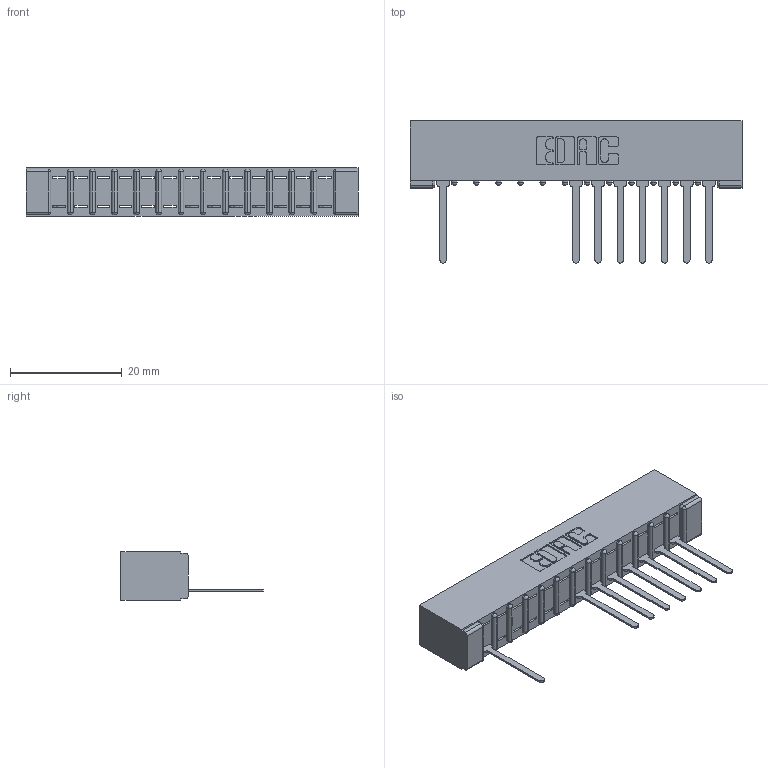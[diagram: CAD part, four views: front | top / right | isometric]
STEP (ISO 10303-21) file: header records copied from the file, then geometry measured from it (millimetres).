
FILE_DESCRIPTION (( 'STEP AP203' ), '1' );
FILE_NAME ('357-013-547-101.STEP', '2018-08-07T22:45:16', ( '' ), ( '' ), 'SwSTEP 2.0', 'SolidWorks 2016', '' );
FILE_SCHEMA (( 'CONFIG_CONTROL_DESIGN' ));
Length unit declared in the file: inch
Products named in the file (3): 307-290-001_547; 357-013-547-101; 307 Part_No Mounting Lugs
Assembly tree (9 placements, depth 2):
  357-013-547-101
    307 Part_No Mounting Lugs
    307-290-001_547  x8
Bounding box: 59.39 x 25.43 x 8.71 mm (x, y, z)
Volume: 3916.4 mm3; surface area: 5715 mm2
Topology: 9 solids, 9 shells, 672 faces, 1915 edges, 1226 vertices
Faces by surface type: plane 422, cylinder 222, sphere 28
Entity records: 14250 total; most frequent: CARTESIAN_POINT 2411, ORIENTED_EDGE 2402, DIRECTION 2355, EDGE_CURVE 1201, VECTOR 911, LINE 911, VERTEX_POINT 778, AXIS2_PLACEMENT_3D 722
